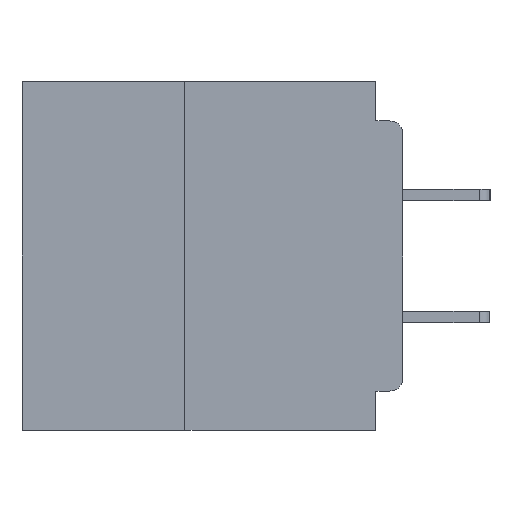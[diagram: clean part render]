
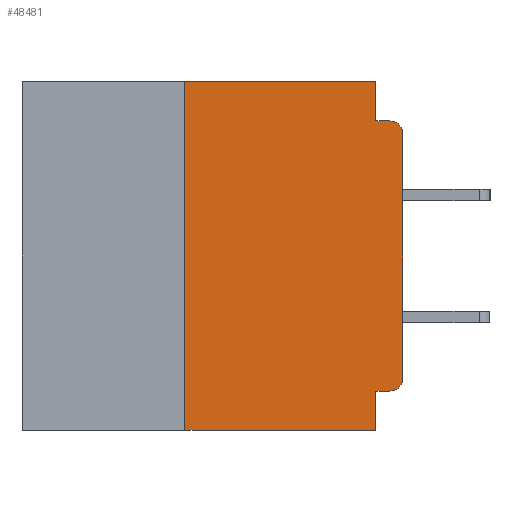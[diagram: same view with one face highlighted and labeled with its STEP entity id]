
A CAD part, left-side view. The second image highlights one B-rep face of the part: STEP entity #48481.
In plain terms, the highlighted planar face has unit normal (-1, 0, 0).
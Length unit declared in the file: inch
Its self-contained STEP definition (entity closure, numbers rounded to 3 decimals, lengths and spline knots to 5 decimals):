
#321 = ORIENTED_EDGE ( 'NONE', *, *, #676, .F. ) ;
#676 = EDGE_CURVE ( 'NONE', #18990, #21128, #39053, .T. ) ;
#1496 = DIRECTION ( 'NONE',  ( 0., 0., 1. ) ) ;
#1643 = ORIENTED_EDGE ( 'NONE', *, *, #28747, .F. ) ;
#3093 = VERTEX_POINT ( 'NONE', #40259 ) ;
#3158 = CARTESIAN_POINT ( 'NONE',  ( 0., 0.015, -0.045 ) ) ;
#3267 = DIRECTION ( 'NONE',  ( 0., -1., 0. ) ) ;
#3418 = EDGE_CURVE ( 'NONE', #25321, #5554, #16932, .T. ) ;
#3849 = EDGE_LOOP ( 'NONE', ( #17737, #19673, #33691, #9773, #321, #1643, #48436, #43773, #50732, #34626 ) ) ;
#4233 = VECTOR ( 'NONE', #39908, 39.37008 ) ;
#4640 = CIRCLE ( 'NONE', #12940, 0.015 ) ;
#5275 = VERTEX_POINT ( 'NONE', #44676 ) ;
#5554 = VERTEX_POINT ( 'NONE', #3158 ) ;
#6239 = DIRECTION ( 'NONE',  ( 0., 0., -1. ) ) ;
#6496 = VERTEX_POINT ( 'NONE', #25127 ) ;
#6820 = VERTEX_POINT ( 'NONE', #15504 ) ;
#6848 = LINE ( 'NONE', #31713, #18690 ) ;
#7762 = VECTOR ( 'NONE', #11895, 39.37008 ) ;
#8221 = VECTOR ( 'NONE', #3267, 39.37008 ) ;
#8631 = VECTOR ( 'NONE', #40986, 39.37008 ) ;
#8964 = LINE ( 'NONE', #28776, #49433 ) ;
#9773 = ORIENTED_EDGE ( 'NONE', *, *, #10796, .F. ) ;
#10038 = CARTESIAN_POINT ( 'NONE',  ( 0., 0.437, 0. ) ) ;
#10796 = EDGE_CURVE ( 'NONE', #21128, #6820, #48274, .T. ) ;
#11895 = DIRECTION ( 'NONE',  ( 0., -1., 0. ) ) ;
#12940 = AXIS2_PLACEMENT_3D ( 'NONE', #45242, #21919, #49176 ) ;
#13888 = EDGE_CURVE ( 'NONE', #5275, #45515, #16016, .T. ) ;
#15504 = CARTESIAN_POINT ( 'NONE',  ( 0., 0.031, -0.045 ) ) ;
#15959 = EDGE_CURVE ( 'NONE', #5275, #3093, #4640, .T. ) ;
#16016 = LINE ( 'NONE', #28154, #4233 ) ;
#16932 = CIRCLE ( 'NONE', #25631, 0.015 ) ;
#17418 = EDGE_CURVE ( 'NONE', #6820, #5554, #37087, .T. ) ;
#17652 = CARTESIAN_POINT ( 'NONE',  ( 0., 0.031, -0.4 ) ) ;
#17737 = ORIENTED_EDGE ( 'NONE', *, *, #21401, .T. ) ;
#18065 = PLANE ( 'NONE',  #29745 ) ;
#18690 = VECTOR ( 'NONE', #35621, 39.37008 ) ;
#18785 = EDGE_CURVE ( 'NONE', #43731, #6496, #6848, .T. ) ;
#18990 = VERTEX_POINT ( 'NONE', #25022 ) ;
#19254 = LINE ( 'NONE', #17652, #8631 ) ;
#19673 = ORIENTED_EDGE ( 'NONE', *, *, #3418, .T. ) ;
#21000 = CARTESIAN_POINT ( 'NONE',  ( 0., 0.031, -0.355 ) ) ;
#21128 = VERTEX_POINT ( 'NONE', #50720 ) ;
#21401 = EDGE_CURVE ( 'NONE', #3093, #25321, #40032, .T. ) ;
#21848 = FACE_OUTER_BOUND ( 'NONE', #3849, .T. ) ;
#21919 = DIRECTION ( 'NONE',  ( -1., 0., 0. ) ) ;
#25022 = CARTESIAN_POINT ( 'NONE',  ( 0., 0.25, 0. ) ) ;
#25127 = CARTESIAN_POINT ( 'NONE',  ( 0., 0.031, -0.4 ) ) ;
#25137 = CARTESIAN_POINT ( 'NONE',  ( 0., 0., 0. ) ) ;
#25321 = VERTEX_POINT ( 'NONE', #43785 ) ;
#25631 = AXIS2_PLACEMENT_3D ( 'NONE', #30482, #30383, #30371 ) ;
#26791 = DIRECTION ( 'NONE',  ( 0., 0., -1. ) ) ;
#26876 = CARTESIAN_POINT ( 'NONE',  ( 0., 0., -0.045 ) ) ;
#28154 = CARTESIAN_POINT ( 'NONE',  ( 0., 0., -0.355 ) ) ;
#28747 = EDGE_CURVE ( 'NONE', #43731, #18990, #8964, .T. ) ;
#28776 = CARTESIAN_POINT ( 'NONE',  ( 0., 0.25, -0.4 ) ) ;
#29745 = AXIS2_PLACEMENT_3D ( 'NONE', #10038, #29816, #6239 ) ;
#29816 = DIRECTION ( 'NONE',  ( 1., 0., 0. ) ) ;
#30371 = DIRECTION ( 'NONE',  ( 0., 0., -1. ) ) ;
#30383 = DIRECTION ( 'NONE',  ( -1., 0., 0. ) ) ;
#30482 = CARTESIAN_POINT ( 'NONE',  ( 0., 0.015, -0.06 ) ) ;
#30933 = VECTOR ( 'NONE', #1496, 39.37008 ) ;
#31713 = CARTESIAN_POINT ( 'NONE',  ( 0., 0.437, -0.4 ) ) ;
#32737 = DIRECTION ( 'NONE',  ( 0., 0., 1. ) ) ;
#33691 = ORIENTED_EDGE ( 'NONE', *, *, #17418, .F. ) ;
#34626 = ORIENTED_EDGE ( 'NONE', *, *, #15959, .T. ) ;
#35621 = DIRECTION ( 'NONE',  ( 0., -1., 0. ) ) ;
#37087 = LINE ( 'NONE', #26876, #8221 ) ;
#38238 = EDGE_CURVE ( 'NONE', #45515, #6496, #19254, .T. ) ;
#39053 = LINE ( 'NONE', #48667, #7762 ) ;
#39908 = DIRECTION ( 'NONE',  ( 0., 1., 0. ) ) ;
#40032 = LINE ( 'NONE', #25137, #30933 ) ;
#40259 = CARTESIAN_POINT ( 'NONE',  ( 0., 0., -0.34 ) ) ;
#40986 = DIRECTION ( 'NONE',  ( 0., 0., -1. ) ) ;
#42308 = CARTESIAN_POINT ( 'NONE',  ( 0., 0.031, 0. ) ) ;
#43731 = VERTEX_POINT ( 'NONE', #47430 ) ;
#43773 = ORIENTED_EDGE ( 'NONE', *, *, #38238, .F. ) ;
#43785 = CARTESIAN_POINT ( 'NONE',  ( 0., 0., -0.06 ) ) ;
#44676 = CARTESIAN_POINT ( 'NONE',  ( 0., 0.015, -0.355 ) ) ;
#45242 = CARTESIAN_POINT ( 'NONE',  ( 0., 0.015, -0.34 ) ) ;
#45515 = VERTEX_POINT ( 'NONE', #21000 ) ;
#47060 = VECTOR ( 'NONE', #26791, 39.37008 ) ;
#47430 = CARTESIAN_POINT ( 'NONE',  ( 0., 0.25, -0.4 ) ) ;
#48274 = LINE ( 'NONE', #42308, #47060 ) ;
#48436 = ORIENTED_EDGE ( 'NONE', *, *, #18785, .T. ) ;
#48481 = ADVANCED_FACE ( 'NONE', ( #21848 ), #18065, .F. ) ;
#48667 = CARTESIAN_POINT ( 'NONE',  ( 0., 0.437, 0. ) ) ;
#49176 = DIRECTION ( 'NONE',  ( 0., 0., -1. ) ) ;
#49433 = VECTOR ( 'NONE', #32737, 39.37008 ) ;
#50720 = CARTESIAN_POINT ( 'NONE',  ( 0., 0.031, 0. ) ) ;
#50732 = ORIENTED_EDGE ( 'NONE', *, *, #13888, .F. ) ;
